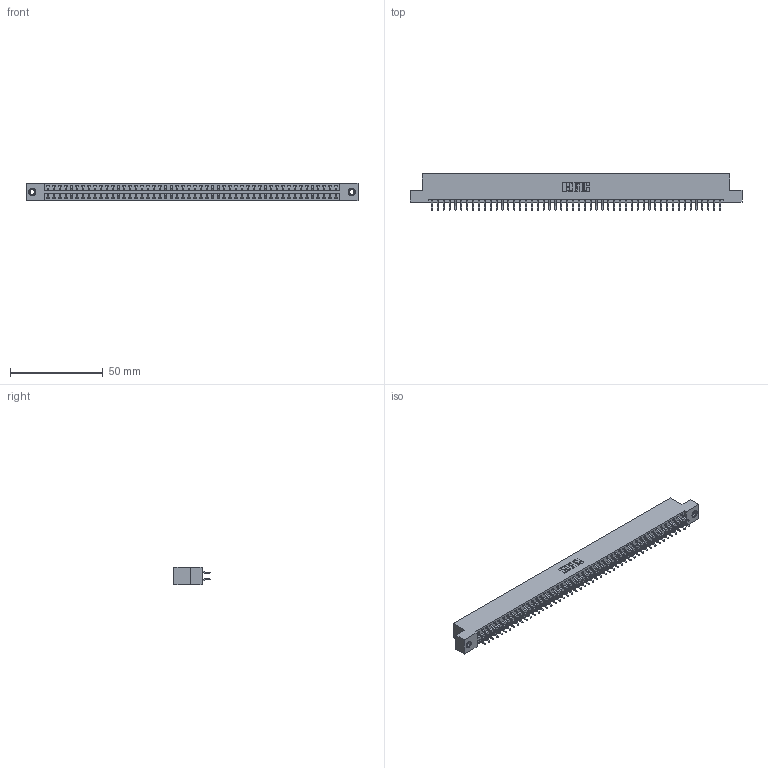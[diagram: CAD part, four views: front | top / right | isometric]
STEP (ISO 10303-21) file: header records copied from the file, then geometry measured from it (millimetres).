
FILE_DESCRIPTION (( 'STEP AP203' ), '1' );
FILE_NAME ('396-100-556-207.STEP', '2019-10-31T05:58:52', ( '' ), ( '' ), 'SwSTEP 2.0', 'SolidWorks 2016', '' );
FILE_SCHEMA (( 'CONFIG_CONTROL_DESIGN' ));
Length unit declared in the file: inch
Products named in the file (4): 345-250-001_345-250-005-103; 345-292-001_556 Tail; 346 Part_Flush Mounting Lugs - 0.156 Dia-TI; 396-100-556-207
Assembly tree (103 placements, depth 2):
  396-100-556-207
    346 Part_Flush Mounting Lugs - 0.156 Dia-TI
    345-292-001_556 Tail  x100
    345-250-001_345-250-005-103  x2
Bounding box: 179.32 x 19.57 x 9.4 mm (x, y, z)
Volume: 17531 mm3; surface area: 24164.1 mm2
Topology: 103 solids, 103 shells, 5982 faces, 17765 edges, 11702 vertices
Faces by surface type: plane 4008, cylinder 1958, cone 12, torus 4
Entity records: 32960 total; most frequent: CARTESIAN_POINT 5419, ORIENTED_EDGE 5334, DIRECTION 4841, EDGE_CURVE 2667, VECTOR 2307, LINE 2307, VERTEX_POINT 1772, AXIS2_PLACEMENT_3D 1267
